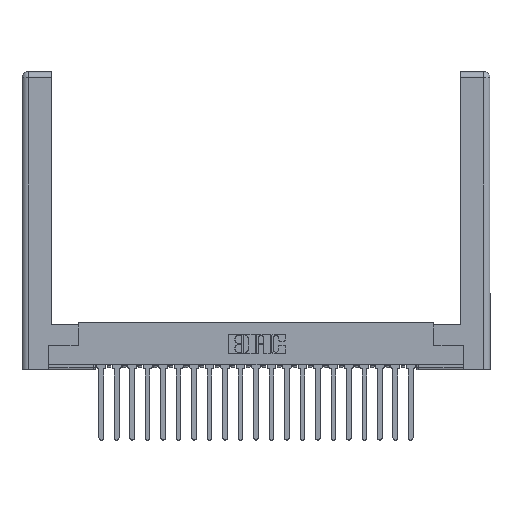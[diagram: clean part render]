
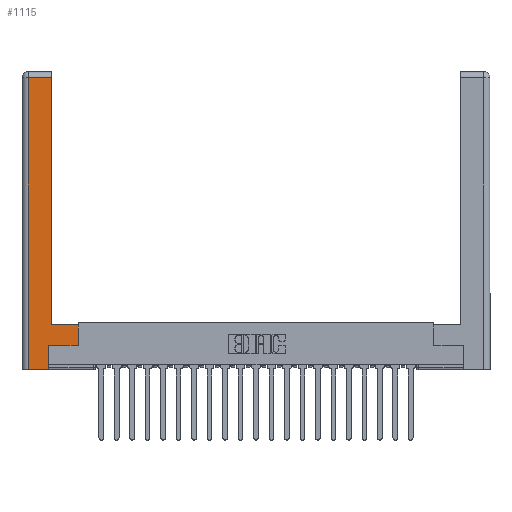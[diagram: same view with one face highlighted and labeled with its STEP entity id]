
A CAD part, top view. The second image highlights one B-rep face of the part: STEP entity #1115.
In plain terms, the highlighted planar face has unit normal (0, 0, 1).
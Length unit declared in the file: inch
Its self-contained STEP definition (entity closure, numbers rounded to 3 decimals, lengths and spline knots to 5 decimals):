
#83 = CARTESIAN_POINT ( 'NONE',  ( 0.265, 0., 0. ) ) ;
#89 = LINE ( 'NONE', #10268, #9298 ) ;
#482 = DIRECTION ( 'NONE',  ( 0., -1., 0. ) ) ;
#615 = EDGE_CURVE ( 'NONE', #9019, #18663, #4217, .T. ) ;
#887 = LINE ( 'NONE', #9185, #20534 ) ;
#1115 = ADVANCED_FACE ( 'NONE', ( #13714 ), #20532, .F. ) ;
#1656 = CARTESIAN_POINT ( 'NONE',  ( 0.265, 0.245, 0. ) ) ;
#2103 = EDGE_CURVE ( 'NONE', #16602, #22294, #19473, .T. ) ;
#2582 = ORIENTED_EDGE ( 'NONE', *, *, #8515, .T. ) ;
#2815 = EDGE_CURVE ( 'NONE', #22294, #17645, #89, .T. ) ;
#2943 = DIRECTION ( 'NONE',  ( 1., 0., 0. ) ) ;
#4217 = LINE ( 'NONE', #7735, #11683 ) ;
#4355 = ORIENTED_EDGE ( 'NONE', *, *, #17845, .T. ) ;
#4857 = EDGE_LOOP ( 'NONE', ( #4921, #6732, #12299, #2582, #21264, #9112, #4355, #10969 ) ) ;
#4921 = ORIENTED_EDGE ( 'NONE', *, *, #7554, .T. ) ;
#5094 = DIRECTION ( 'NONE',  ( 0., 1., 0. ) ) ;
#5444 = CARTESIAN_POINT ( 'NONE',  ( 0.295, 0.45, 0. ) ) ;
#6732 = ORIENTED_EDGE ( 'NONE', *, *, #615, .T. ) ;
#7554 = EDGE_CURVE ( 'NONE', #8205, #9019, #17693, .T. ) ;
#7735 = CARTESIAN_POINT ( 'NONE',  ( 0.0615, 2.94, 0. ) ) ;
#7822 = DIRECTION ( 'NONE',  ( -1., 0., 0. ) ) ;
#8205 = VERTEX_POINT ( 'NONE', #23096 ) ;
#8213 = VECTOR ( 'NONE', #482, 39.37008 ) ;
#8515 = EDGE_CURVE ( 'NONE', #12465, #16602, #887, .T. ) ;
#8928 = LINE ( 'NONE', #5444, #21681 ) ;
#9019 = VERTEX_POINT ( 'NONE', #14343 ) ;
#9112 = ORIENTED_EDGE ( 'NONE', *, *, #2815, .T. ) ;
#9185 = CARTESIAN_POINT ( 'NONE',  ( 0.265, 0., 0. ) ) ;
#9298 = VECTOR ( 'NONE', #2943, 39.37008 ) ;
#9541 = CARTESIAN_POINT ( 'NONE',  ( 0.0615, 0., 0. ) ) ;
#9837 = CARTESIAN_POINT ( 'NONE',  ( 0.0615, 0., 0. ) ) ;
#10268 = CARTESIAN_POINT ( 'NONE',  ( 0.565, 0.245, 0. ) ) ;
#10770 = EDGE_CURVE ( 'NONE', #18663, #12465, #23839, .T. ) ;
#10969 = ORIENTED_EDGE ( 'NONE', *, *, #19345, .T. ) ;
#11349 = DIRECTION ( 'NONE',  ( -1., 0., 0. ) ) ;
#11683 = VECTOR ( 'NONE', #7822, 39.37008 ) ;
#12299 = ORIENTED_EDGE ( 'NONE', *, *, #10770, .T. ) ;
#12465 = VERTEX_POINT ( 'NONE', #9541 ) ;
#12743 = DIRECTION ( 'NONE',  ( 0., 1., 0. ) ) ;
#13658 = VECTOR ( 'NONE', #5094, 39.37008 ) ;
#13714 = FACE_OUTER_BOUND ( 'NONE', #4857, .T. ) ;
#14343 = CARTESIAN_POINT ( 'NONE',  ( 0.295, 2.94, 0. ) ) ;
#14585 = DIRECTION ( 'NONE',  ( -1., 0., 0. ) ) ;
#14615 = VERTEX_POINT ( 'NONE', #23463 ) ;
#14617 = CARTESIAN_POINT ( 'NONE',  ( 0.0615, 2.94, 0. ) ) ;
#14772 = CARTESIAN_POINT ( 'NONE',  ( 0.295, 3., 0. ) ) ;
#15989 = VECTOR ( 'NONE', #12743, 39.37008 ) ;
#16556 = DIRECTION ( 'NONE',  ( 1., 0., 0. ) ) ;
#16602 = VERTEX_POINT ( 'NONE', #83 ) ;
#16877 = DIRECTION ( 'NONE',  ( 0., 1., 0. ) ) ;
#17093 = CARTESIAN_POINT ( 'NONE',  ( 0.565, 0.245, 0. ) ) ;
#17211 = CARTESIAN_POINT ( 'NONE',  ( 0., 0., 0. ) ) ;
#17645 = VERTEX_POINT ( 'NONE', #17093 ) ;
#17693 = LINE ( 'NONE', #14772, #22589 ) ;
#17845 = EDGE_CURVE ( 'NONE', #17645, #14615, #19459, .T. ) ;
#18039 = AXIS2_PLACEMENT_3D ( 'NONE', #17211, #22516, #11349 ) ;
#18663 = VERTEX_POINT ( 'NONE', #14617 ) ;
#19225 = CARTESIAN_POINT ( 'NONE',  ( 0.265, 0.245, 0. ) ) ;
#19345 = EDGE_CURVE ( 'NONE', #14615, #8205, #8928, .T. ) ;
#19459 = LINE ( 'NONE', #23346, #13658 ) ;
#19473 = LINE ( 'NONE', #1656, #15989 ) ;
#20532 = PLANE ( 'NONE',  #18039 ) ;
#20534 = VECTOR ( 'NONE', #16556, 39.37008 ) ;
#21264 = ORIENTED_EDGE ( 'NONE', *, *, #2103, .T. ) ;
#21681 = VECTOR ( 'NONE', #14585, 39.37008 ) ;
#22294 = VERTEX_POINT ( 'NONE', #19225 ) ;
#22516 = DIRECTION ( 'NONE',  ( 0., 0., -1. ) ) ;
#22589 = VECTOR ( 'NONE', #16877, 39.37008 ) ;
#23096 = CARTESIAN_POINT ( 'NONE',  ( 0.295, 0.45, 0. ) ) ;
#23346 = CARTESIAN_POINT ( 'NONE',  ( 0.565, 0.45, 0. ) ) ;
#23463 = CARTESIAN_POINT ( 'NONE',  ( 0.565, 0.45, 0. ) ) ;
#23839 = LINE ( 'NONE', #9837, #8213 ) ;
